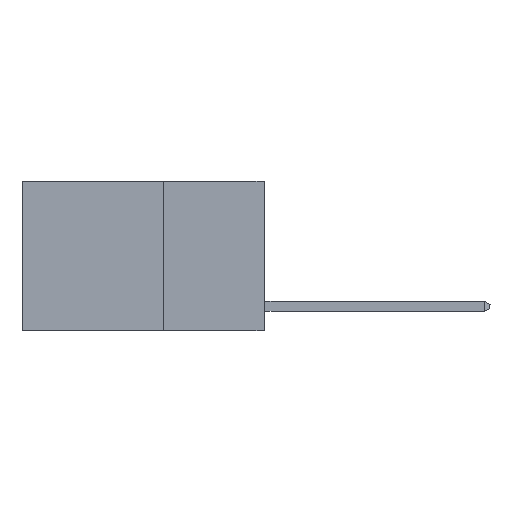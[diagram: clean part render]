
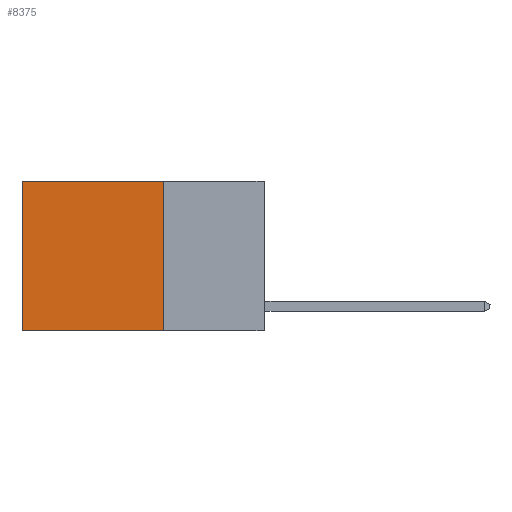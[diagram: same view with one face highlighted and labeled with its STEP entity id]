
A CAD part, left-side view. The second image highlights one B-rep face of the part: STEP entity #8375.
In plain terms, the highlighted planar face has unit normal (-1, 0, 0).
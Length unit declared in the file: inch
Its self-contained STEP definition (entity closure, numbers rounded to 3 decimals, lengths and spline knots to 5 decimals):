
#90 = CARTESIAN_POINT ( 'NONE',  ( 0.2625, 0.25, -0.37 ) ) ;
#226 = VECTOR ( 'NONE', #9541, 39.37008 ) ;
#300 = VERTEX_POINT ( 'NONE', #2701 ) ;
#968 = CARTESIAN_POINT ( 'NONE',  ( 0.2625, 0.25, 0. ) ) ;
#1722 = CARTESIAN_POINT ( 'NONE',  ( 0.2625, 0.25, 0. ) ) ;
#2010 = LINE ( 'NONE', #10490, #226 ) ;
#2526 = EDGE_CURVE ( 'NONE', #10776, #2692, #10329, .T. ) ;
#2692 = VERTEX_POINT ( 'NONE', #90 ) ;
#2701 = CARTESIAN_POINT ( 'NONE',  ( 0.2625, 0.6, -0.37 ) ) ;
#3022 = VECTOR ( 'NONE', #5557, 39.37008 ) ;
#3286 = PLANE ( 'NONE',  #7202 ) ;
#3970 = FACE_OUTER_BOUND ( 'NONE', #10071, .T. ) ;
#4044 = DIRECTION ( 'NONE',  ( 1., 0., 0. ) ) ;
#4156 = DIRECTION ( 'NONE',  ( 0., 0., -1. ) ) ;
#4203 = ORIENTED_EDGE ( 'NONE', *, *, #2526, .F. ) ;
#4484 = ORIENTED_EDGE ( 'NONE', *, *, #9881, .T. ) ;
#5557 = DIRECTION ( 'NONE',  ( 0., 0., -1. ) ) ;
#5700 = ORIENTED_EDGE ( 'NONE', *, *, #6916, .F. ) ;
#6726 = LINE ( 'NONE', #7803, #7254 ) ;
#6876 = CARTESIAN_POINT ( 'NONE',  ( 0.2625, 0.25, -0.37 ) ) ;
#6916 = EDGE_CURVE ( 'NONE', #2692, #300, #8014, .T. ) ;
#7202 = AXIS2_PLACEMENT_3D ( 'NONE', #11859, #4044, #4156 ) ;
#7254 = VECTOR ( 'NONE', #10560, 39.37008 ) ;
#7803 = CARTESIAN_POINT ( 'NONE',  ( 0.2625, 0.25, 0. ) ) ;
#8014 = LINE ( 'NONE', #6876, #11625 ) ;
#8375 = ADVANCED_FACE ( 'NONE', ( #3970 ), #3286, .F. ) ;
#9541 = DIRECTION ( 'NONE',  ( 0., 0., -1. ) ) ;
#9831 = CARTESIAN_POINT ( 'NONE',  ( 0.2625, 0.6, 0. ) ) ;
#9881 = EDGE_CURVE ( 'NONE', #11983, #300, #2010, .T. ) ;
#10071 = EDGE_LOOP ( 'NONE', ( #4484, #5700, #4203, #10269 ) ) ;
#10269 = ORIENTED_EDGE ( 'NONE', *, *, #10804, .T. ) ;
#10329 = LINE ( 'NONE', #1722, #3022 ) ;
#10490 = CARTESIAN_POINT ( 'NONE',  ( 0.2625, 0.6, 0. ) ) ;
#10560 = DIRECTION ( 'NONE',  ( 0., 1., 0. ) ) ;
#10764 = DIRECTION ( 'NONE',  ( 0., 1., 0. ) ) ;
#10776 = VERTEX_POINT ( 'NONE', #968 ) ;
#10804 = EDGE_CURVE ( 'NONE', #10776, #11983, #6726, .T. ) ;
#11625 = VECTOR ( 'NONE', #10764, 39.37008 ) ;
#11859 = CARTESIAN_POINT ( 'NONE',  ( 0.2625, 0.25, 0. ) ) ;
#11983 = VERTEX_POINT ( 'NONE', #9831 ) ;
